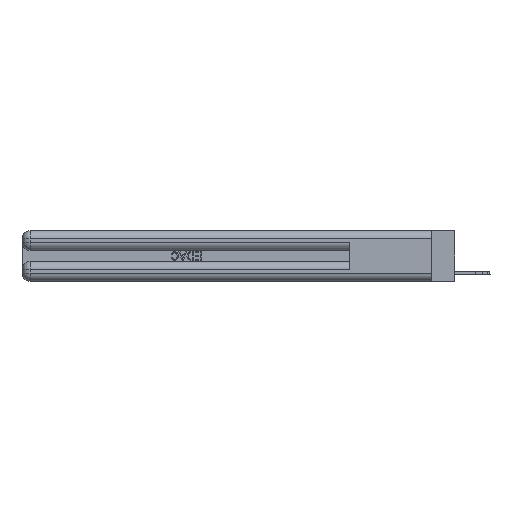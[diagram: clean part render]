
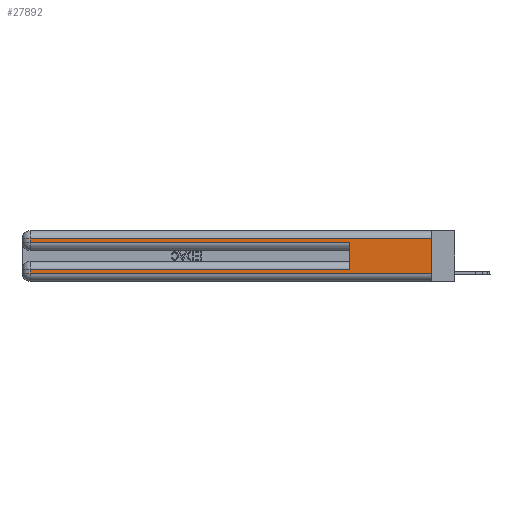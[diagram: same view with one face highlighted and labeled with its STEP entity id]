
A CAD part, left-side view. The second image highlights one B-rep face of the part: STEP entity #27892.
In plain terms, the highlighted planar face has unit normal (-1, 0, 0).
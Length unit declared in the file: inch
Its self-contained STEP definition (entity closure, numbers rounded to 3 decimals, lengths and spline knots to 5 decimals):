
#1170 = PLANE ( 'NONE',  #28021 ) ;
#1470 = VECTOR ( 'NONE', #16240, 39.37008 ) ;
#1692 = ORIENTED_EDGE ( 'NONE', *, *, #20078, .T. ) ;
#1699 = VERTEX_POINT ( 'NONE', #14079 ) ;
#2060 = CARTESIAN_POINT ( 'NONE',  ( 0., 0., 0.085 ) ) ;
#3196 = EDGE_CURVE ( 'NONE', #17519, #6363, #7809, .T. ) ;
#3236 = EDGE_CURVE ( 'NONE', #16245, #1699, #15190, .T. ) ;
#3630 = CARTESIAN_POINT ( 'NONE',  ( 0., 0., 0.06 ) ) ;
#4670 = CARTESIAN_POINT ( 'NONE',  ( 0., 0.6, 0.285 ) ) ;
#4677 = CARTESIAN_POINT ( 'NONE',  ( 0., 2.94, 0.37 ) ) ;
#4907 = EDGE_CURVE ( 'NONE', #1699, #6363, #15772, .T. ) ;
#5214 = ORIENTED_EDGE ( 'NONE', *, *, #27030, .T. ) ;
#5712 = ORIENTED_EDGE ( 'NONE', *, *, #4907, .T. ) ;
#6363 = VERTEX_POINT ( 'NONE', #20848 ) ;
#7809 = LINE ( 'NONE', #19355, #24787 ) ;
#7997 = VECTOR ( 'NONE', #27847, 39.37008 ) ;
#8676 = LINE ( 'NONE', #2060, #7997 ) ;
#8701 = DIRECTION ( 'NONE',  ( 0., -1., 0. ) ) ;
#8926 = ORIENTED_EDGE ( 'NONE', *, *, #16047, .T. ) ;
#9289 = VERTEX_POINT ( 'NONE', #4670 ) ;
#11066 = DIRECTION ( 'NONE',  ( 0., 1., 0. ) ) ;
#11117 = CARTESIAN_POINT ( 'NONE',  ( 0., 0., 0.31 ) ) ;
#11694 = VERTEX_POINT ( 'NONE', #20618 ) ;
#11768 = CARTESIAN_POINT ( 'NONE',  ( 0., 0.6, 0.145 ) ) ;
#12232 = CARTESIAN_POINT ( 'NONE',  ( 0., 2.94, 0.31 ) ) ;
#12341 = DIRECTION ( 'NONE',  ( 0., -1., 0. ) ) ;
#12458 = EDGE_CURVE ( 'NONE', #17237, #11694, #13875, .T. ) ;
#12944 = LINE ( 'NONE', #29347, #17246 ) ;
#13153 = ORIENTED_EDGE ( 'NONE', *, *, #3196, .F. ) ;
#13875 = LINE ( 'NONE', #4677, #24623 ) ;
#13946 = ORIENTED_EDGE ( 'NONE', *, *, #3236, .T. ) ;
#14079 = CARTESIAN_POINT ( 'NONE',  ( 0., 2.94, 0.06 ) ) ;
#15190 = LINE ( 'NONE', #29876, #19386 ) ;
#15772 = LINE ( 'NONE', #3630, #21361 ) ;
#16047 = EDGE_CURVE ( 'NONE', #25064, #16245, #8676, .T. ) ;
#16086 = LINE ( 'NONE', #11768, #1470 ) ;
#16240 = DIRECTION ( 'NONE',  ( 0., 0., 1. ) ) ;
#16245 = VERTEX_POINT ( 'NONE', #26764 ) ;
#16512 = DIRECTION ( 'NONE',  ( 0., 0., -1. ) ) ;
#16861 = CARTESIAN_POINT ( 'NONE',  ( 0., 0.6, 0.085 ) ) ;
#17237 = VERTEX_POINT ( 'NONE', #12232 ) ;
#17246 = VECTOR ( 'NONE', #12341, 39.37008 ) ;
#17519 = VERTEX_POINT ( 'NONE', #11117 ) ;
#17625 = CARTESIAN_POINT ( 'NONE',  ( 0., 0., 0.37 ) ) ;
#19355 = CARTESIAN_POINT ( 'NONE',  ( 0., 0., 0.37 ) ) ;
#19386 = VECTOR ( 'NONE', #26853, 39.37008 ) ;
#19919 = DIRECTION ( 'NONE',  ( 0., 0., -1. ) ) ;
#20001 = VECTOR ( 'NONE', #11066, 39.37008 ) ;
#20078 = EDGE_CURVE ( 'NONE', #17519, #17237, #25354, .T. ) ;
#20272 = ORIENTED_EDGE ( 'NONE', *, *, #12458, .T. ) ;
#20618 = CARTESIAN_POINT ( 'NONE',  ( 0., 2.94, 0.285 ) ) ;
#20848 = CARTESIAN_POINT ( 'NONE',  ( 0., 0., 0.06 ) ) ;
#21361 = VECTOR ( 'NONE', #8701, 39.37008 ) ;
#22601 = EDGE_CURVE ( 'NONE', #25064, #9289, #16086, .T. ) ;
#22716 = EDGE_LOOP ( 'NONE', ( #13153, #1692, #20272, #5214, #24419, #8926, #13946, #5712 ) ) ;
#22745 = CARTESIAN_POINT ( 'NONE',  ( 0., 0., 0.31 ) ) ;
#24419 = ORIENTED_EDGE ( 'NONE', *, *, #22601, .F. ) ;
#24623 = VECTOR ( 'NONE', #16512, 39.37008 ) ;
#24787 = VECTOR ( 'NONE', #26708, 39.37008 ) ;
#25064 = VERTEX_POINT ( 'NONE', #16861 ) ;
#25354 = LINE ( 'NONE', #22745, #20001 ) ;
#26708 = DIRECTION ( 'NONE',  ( 0., 0., -1. ) ) ;
#26764 = CARTESIAN_POINT ( 'NONE',  ( 0., 2.94, 0.085 ) ) ;
#26853 = DIRECTION ( 'NONE',  ( 0., 0., -1. ) ) ;
#27030 = EDGE_CURVE ( 'NONE', #11694, #9289, #12944, .T. ) ;
#27847 = DIRECTION ( 'NONE',  ( 0., 1., 0. ) ) ;
#27892 = ADVANCED_FACE ( 'NONE', ( #29101 ), #1170, .F. ) ;
#28021 = AXIS2_PLACEMENT_3D ( 'NONE', #17625, #29544, #19919 ) ;
#29101 = FACE_OUTER_BOUND ( 'NONE', #22716, .T. ) ;
#29347 = CARTESIAN_POINT ( 'NONE',  ( 0., 0., 0.285 ) ) ;
#29544 = DIRECTION ( 'NONE',  ( 1., 0., 0. ) ) ;
#29876 = CARTESIAN_POINT ( 'NONE',  ( 0., 2.94, 0.37 ) ) ;
